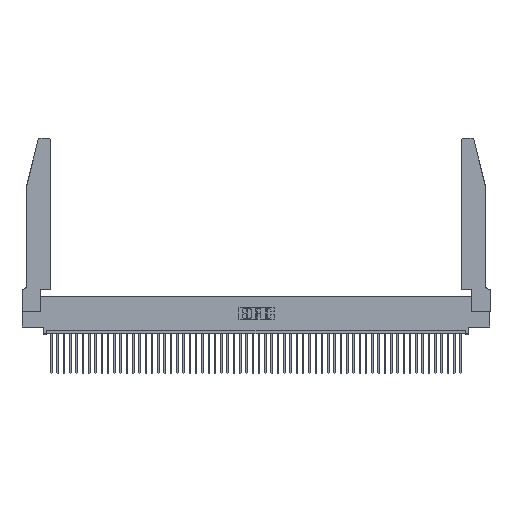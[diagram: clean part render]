
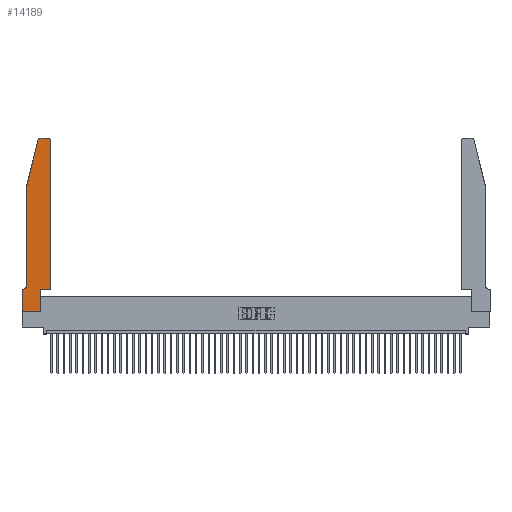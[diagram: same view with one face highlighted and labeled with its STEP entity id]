
A CAD part, top view. The second image highlights one B-rep face of the part: STEP entity #14189.
In plain terms, the highlighted planar face has unit normal (0, 0, 1).
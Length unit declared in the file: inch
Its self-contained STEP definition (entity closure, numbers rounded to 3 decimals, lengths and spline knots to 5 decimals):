
#251 = LINE ( 'NONE', #29298, #12018 ) ;
#437 = ORIENTED_EDGE ( 'NONE', *, *, #23361, .T. ) ;
#766 = CARTESIAN_POINT ( 'NONE',  ( 0., 0.35, 0.37 ) ) ;
#1312 = AXIS2_PLACEMENT_3D ( 'NONE', #18768, #46445, #26723 ) ;
#1600 = DIRECTION ( 'NONE',  ( 1., 0., 0. ) ) ;
#1674 = CARTESIAN_POINT ( 'NONE',  ( 0.4505, 0.35, 0.37 ) ) ;
#3742 = VERTEX_POINT ( 'NONE', #34626 ) ;
#4848 = CARTESIAN_POINT ( 'NONE',  ( 0.0055, 0.42, 0.37 ) ) ;
#5024 = DIRECTION ( 'NONE',  ( -1., 0., 0. ) ) ;
#5500 = EDGE_CURVE ( 'NONE', #7361, #27276, #27126, .T. ) ;
#5627 = VECTOR ( 'NONE', #22442, 39.37008 ) ;
#6655 = VERTEX_POINT ( 'NONE', #37161 ) ;
#6706 = ORIENTED_EDGE ( 'NONE', *, *, #20471, .T. ) ;
#7361 = VERTEX_POINT ( 'NONE', #25084 ) ;
#7754 = EDGE_CURVE ( 'NONE', #38501, #39124, #31953, .T. ) ;
#8477 = LINE ( 'NONE', #25552, #33258 ) ;
#9182 = CARTESIAN_POINT ( 'NONE',  ( 0.0755, 2., 0.37 ) ) ;
#10117 = ORIENTED_EDGE ( 'NONE', *, *, #37200, .T. ) ;
#10160 = EDGE_CURVE ( 'NONE', #29667, #31618, #251, .T. ) ;
#10654 = CIRCLE ( 'NONE', #1312, 0.03 ) ;
#10941 = CARTESIAN_POINT ( 'NONE',  ( 0.4505, 0.35, 0.37 ) ) ;
#11250 = LINE ( 'NONE', #18465, #5627 ) ;
#11787 = CARTESIAN_POINT ( 'NONE',  ( 0.4505, 2.72, 0.37 ) ) ;
#12018 = VECTOR ( 'NONE', #14263, 39.37008 ) ;
#12628 = VECTOR ( 'NONE', #29541, 39.37008 ) ;
#13514 = DIRECTION ( 'NONE',  ( 1., 0., 0. ) ) ;
#13837 = EDGE_CURVE ( 'NONE', #3742, #39941, #11250, .T. ) ;
#14189 = ADVANCED_FACE ( 'NONE', ( #18040 ), #33771, .T. ) ;
#14263 = DIRECTION ( 'NONE',  ( -1., 0., 0. ) ) ;
#14275 = LINE ( 'NONE', #9182, #50904 ) ;
#14694 = EDGE_CURVE ( 'NONE', #39941, #50502, #14275, .T. ) ;
#14888 = ORIENTED_EDGE ( 'NONE', *, *, #10160, .T. ) ;
#15556 = VERTEX_POINT ( 'NONE', #20622 ) ;
#15825 = CARTESIAN_POINT ( 'NONE',  ( 0.4205, 2.75, 0.37 ) ) ;
#17149 = CARTESIAN_POINT ( 'NONE',  ( 0.0755, 2., 0.37 ) ) ;
#17586 = CARTESIAN_POINT ( 'NONE',  ( 0.2865, 0., 0.37 ) ) ;
#18040 = FACE_OUTER_BOUND ( 'NONE', #24600, .T. ) ;
#18465 = CARTESIAN_POINT ( 'NONE',  ( 0.0755, 2., 0.37 ) ) ;
#18768 = CARTESIAN_POINT ( 'NONE',  ( 0.284, 2.72, 0.37 ) ) ;
#19787 = EDGE_CURVE ( 'NONE', #15556, #3742, #10654, .T. ) ;
#20448 = CARTESIAN_POINT ( 'NONE',  ( 0.4205, 2.72, 0.37 ) ) ;
#20471 = EDGE_CURVE ( 'NONE', #39124, #48306, #49274, .T. ) ;
#20622 = CARTESIAN_POINT ( 'NONE',  ( 0.284, 2.75, 0.37 ) ) ;
#21075 = DIRECTION ( 'NONE',  ( 1., 0., 0. ) ) ;
#21123 = VECTOR ( 'NONE', #30496, 39.37008 ) ;
#21425 = ORIENTED_EDGE ( 'NONE', *, *, #7754, .T. ) ;
#21516 = AXIS2_PLACEMENT_3D ( 'NONE', #4848, #36578, #5024 ) ;
#21741 = DIRECTION ( 'NONE',  ( -1., 0., 0. ) ) ;
#21933 = DIRECTION ( 'NONE',  ( 0., 1., 0. ) ) ;
#22178 = VECTOR ( 'NONE', #21075, 39.37008 ) ;
#22442 = DIRECTION ( 'NONE',  ( -0.239, -0.971, 0. ) ) ;
#23361 = EDGE_CURVE ( 'NONE', #31618, #7361, #50341, .T. ) ;
#23922 = ORIENTED_EDGE ( 'NONE', *, *, #5500, .T. ) ;
#24600 = EDGE_LOOP ( 'NONE', ( #10117, #33265, #48414, #45579, #25242, #14888, #437, #23922, #29068, #45466, #21425, #6706 ) ) ;
#25084 = CARTESIAN_POINT ( 'NONE',  ( 0., 0., 0.37 ) ) ;
#25242 = ORIENTED_EDGE ( 'NONE', *, *, #28977, .T. ) ;
#25552 = CARTESIAN_POINT ( 'NONE',  ( 0.2865, 0.35, 0.37 ) ) ;
#25659 = DIRECTION ( 'NONE',  ( 0., 0., 1. ) ) ;
#25872 = CIRCLE ( 'NONE', #21516, 0.07 ) ;
#26298 = CARTESIAN_POINT ( 'NONE',  ( 0.0055, 0.35, 0.37 ) ) ;
#26723 = DIRECTION ( 'NONE',  ( 1., 0., 0. ) ) ;
#27126 = LINE ( 'NONE', #49386, #33261 ) ;
#27276 = VERTEX_POINT ( 'NONE', #17586 ) ;
#28254 = DIRECTION ( 'NONE',  ( 0., 0., 1. ) ) ;
#28977 = EDGE_CURVE ( 'NONE', #50502, #29667, #25872, .T. ) ;
#29068 = ORIENTED_EDGE ( 'NONE', *, *, #37250, .T. ) ;
#29298 = CARTESIAN_POINT ( 'NONE',  ( 0.0755, 0.35, 0.37 ) ) ;
#29541 = DIRECTION ( 'NONE',  ( 0., 1., 0. ) ) ;
#29667 = VERTEX_POINT ( 'NONE', #26298 ) ;
#30496 = DIRECTION ( 'NONE',  ( 0., -1., 0. ) ) ;
#31618 = VERTEX_POINT ( 'NONE', #766 ) ;
#31953 = LINE ( 'NONE', #1674, #12628 ) ;
#32299 = AXIS2_PLACEMENT_3D ( 'NONE', #49227, #25659, #1600 ) ;
#33258 = VECTOR ( 'NONE', #21933, 39.37008 ) ;
#33261 = VECTOR ( 'NONE', #13514, 39.37008 ) ;
#33265 = ORIENTED_EDGE ( 'NONE', *, *, #19787, .T. ) ;
#33771 = PLANE ( 'NONE',  #32299 ) ;
#33869 = LINE ( 'NONE', #44546, #45657 ) ;
#34448 = CARTESIAN_POINT ( 'NONE',  ( 0., 0., 0.37 ) ) ;
#34482 = DIRECTION ( 'NONE',  ( 0., -1., 0. ) ) ;
#34626 = CARTESIAN_POINT ( 'NONE',  ( 0.25487, 2.72718, 0.37 ) ) ;
#36578 = DIRECTION ( 'NONE',  ( 0., 0., -1. ) ) ;
#36832 = CARTESIAN_POINT ( 'NONE',  ( 0.4505, 0.35, 0.37 ) ) ;
#37161 = CARTESIAN_POINT ( 'NONE',  ( 0.2865, 0.35, 0.37 ) ) ;
#37200 = EDGE_CURVE ( 'NONE', #48306, #15556, #33869, .T. ) ;
#37250 = EDGE_CURVE ( 'NONE', #27276, #6655, #8477, .T. ) ;
#38501 = VERTEX_POINT ( 'NONE', #10941 ) ;
#39124 = VERTEX_POINT ( 'NONE', #11787 ) ;
#39941 = VERTEX_POINT ( 'NONE', #17149 ) ;
#40783 = AXIS2_PLACEMENT_3D ( 'NONE', #20448, #28254, #48162 ) ;
#41342 = LINE ( 'NONE', #36832, #22178 ) ;
#41473 = CARTESIAN_POINT ( 'NONE',  ( 0.0755, 0.42, 0.37 ) ) ;
#44546 = CARTESIAN_POINT ( 'NONE',  ( 0.2605, 2.75, 0.37 ) ) ;
#45466 = ORIENTED_EDGE ( 'NONE', *, *, #50231, .T. ) ;
#45579 = ORIENTED_EDGE ( 'NONE', *, *, #14694, .T. ) ;
#45657 = VECTOR ( 'NONE', #21741, 39.37008 ) ;
#46445 = DIRECTION ( 'NONE',  ( 0., 0., 1. ) ) ;
#48162 = DIRECTION ( 'NONE',  ( 1., 0., 0. ) ) ;
#48306 = VERTEX_POINT ( 'NONE', #15825 ) ;
#48414 = ORIENTED_EDGE ( 'NONE', *, *, #13837, .T. ) ;
#49227 = CARTESIAN_POINT ( 'NONE',  ( 0., 0.35, 0.37 ) ) ;
#49274 = CIRCLE ( 'NONE', #40783, 0.03 ) ;
#49386 = CARTESIAN_POINT ( 'NONE',  ( 0., 0., 0.37 ) ) ;
#50231 = EDGE_CURVE ( 'NONE', #6655, #38501, #41342, .T. ) ;
#50341 = LINE ( 'NONE', #34448, #21123 ) ;
#50502 = VERTEX_POINT ( 'NONE', #41473 ) ;
#50904 = VECTOR ( 'NONE', #34482, 39.37008 ) ;
